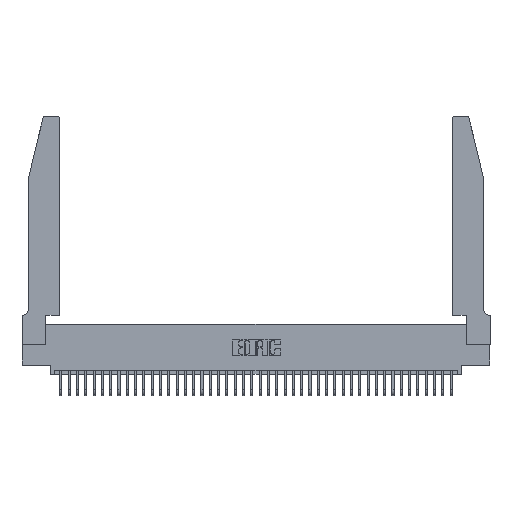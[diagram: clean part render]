
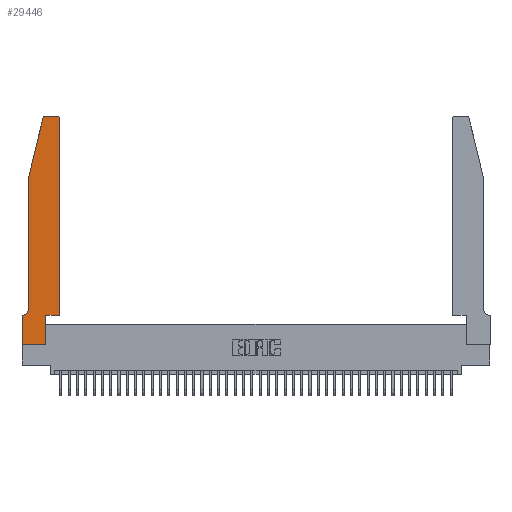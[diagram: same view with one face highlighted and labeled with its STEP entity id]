
A CAD part, top view. The second image highlights one B-rep face of the part: STEP entity #29446.
In plain terms, the highlighted planar face has unit normal (0, 0, 1).
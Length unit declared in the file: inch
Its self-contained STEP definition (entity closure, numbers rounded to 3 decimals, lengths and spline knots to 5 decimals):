
#375 = AXIS2_PLACEMENT_3D ( 'NONE', #7597, #30998, #10996 ) ;
#443 = VERTEX_POINT ( 'NONE', #25061 ) ;
#1392 = CIRCLE ( 'NONE', #7124, 0.03 ) ;
#1863 = ORIENTED_EDGE ( 'NONE', *, *, #19741, .T. ) ;
#1876 = FACE_OUTER_BOUND ( 'NONE', #27281, .T. ) ;
#3593 = LINE ( 'NONE', #36988, #31381 ) ;
#3890 = VECTOR ( 'NONE', #8353, 39.37008 ) ;
#4592 = CARTESIAN_POINT ( 'NONE',  ( 0.284, 2.75, 0.37 ) ) ;
#4842 = EDGE_CURVE ( 'NONE', #22858, #41574, #39534, .T. ) ;
#6413 = VECTOR ( 'NONE', #42172, 39.37008 ) ;
#7063 = ORIENTED_EDGE ( 'NONE', *, *, #30207, .T. ) ;
#7124 = AXIS2_PLACEMENT_3D ( 'NONE', #10562, #33948, #13940 ) ;
#7597 = CARTESIAN_POINT ( 'NONE',  ( 0.0055, 0.42, 0.37 ) ) ;
#8353 = DIRECTION ( 'NONE',  ( -0.239, -0.971, 0. ) ) ;
#8403 = DIRECTION ( 'NONE',  ( 0., 1., 0. ) ) ;
#8424 = DIRECTION ( 'NONE',  ( 0., -1., 0. ) ) ;
#9290 = CARTESIAN_POINT ( 'NONE',  ( 0., 0.35, 0.37 ) ) ;
#9339 = EDGE_CURVE ( 'NONE', #443, #17640, #28686, .T. ) ;
#10196 = VERTEX_POINT ( 'NONE', #34049 ) ;
#10318 = CARTESIAN_POINT ( 'NONE',  ( 0.284, 2.72, 0.37 ) ) ;
#10562 = CARTESIAN_POINT ( 'NONE',  ( 0.4205, 2.72, 0.37 ) ) ;
#10727 = CARTESIAN_POINT ( 'NONE',  ( 0., 0., 0.37 ) ) ;
#10894 = VECTOR ( 'NONE', #42439, 39.37008 ) ;
#10996 = DIRECTION ( 'NONE',  ( -1., 0., 0. ) ) ;
#12201 = DIRECTION ( 'NONE',  ( 1., 0., 0. ) ) ;
#13354 = ORIENTED_EDGE ( 'NONE', *, *, #23397, .T. ) ;
#13368 = LINE ( 'NONE', #19844, #20181 ) ;
#13381 = VERTEX_POINT ( 'NONE', #36469 ) ;
#13696 = DIRECTION ( 'NONE',  ( 1., 0., 0. ) ) ;
#13940 = DIRECTION ( 'NONE',  ( 1., 0., 0. ) ) ;
#14073 = ORIENTED_EDGE ( 'NONE', *, *, #34674, .T. ) ;
#15344 = EDGE_CURVE ( 'NONE', #24610, #22028, #13368, .T. ) ;
#15837 = ORIENTED_EDGE ( 'NONE', *, *, #17032, .T. ) ;
#16259 = VECTOR ( 'NONE', #12201, 39.37008 ) ;
#16424 = DIRECTION ( 'NONE',  ( 0., 0., 1. ) ) ;
#16578 = VERTEX_POINT ( 'NONE', #43088 ) ;
#17032 = EDGE_CURVE ( 'NONE', #41574, #16578, #24220, .T. ) ;
#17319 = LINE ( 'NONE', #22134, #16259 ) ;
#17443 = CIRCLE ( 'NONE', #375, 0.07 ) ;
#17640 = VERTEX_POINT ( 'NONE', #9290 ) ;
#19472 = EDGE_CURVE ( 'NONE', #10196, #42758, #27251, .T. ) ;
#19741 = EDGE_CURVE ( 'NONE', #40538, #22858, #34519, .T. ) ;
#19765 = CARTESIAN_POINT ( 'NONE',  ( 0.4505, 2.72, 0.37 ) ) ;
#19844 = CARTESIAN_POINT ( 'NONE',  ( 0.4505, 0.35, 0.37 ) ) ;
#20168 = DIRECTION ( 'NONE',  ( -1., 0., 0. ) ) ;
#20181 = VECTOR ( 'NONE', #36484, 39.37008 ) ;
#20415 = EDGE_CURVE ( 'NONE', #22028, #13381, #1392, .T. ) ;
#22028 = VERTEX_POINT ( 'NONE', #19765 ) ;
#22134 = CARTESIAN_POINT ( 'NONE',  ( 0., 0., 0.37 ) ) ;
#22150 = CARTESIAN_POINT ( 'NONE',  ( 0.0755, 2., 0.37 ) ) ;
#22830 = VECTOR ( 'NONE', #20168, 39.37008 ) ;
#22858 = VERTEX_POINT ( 'NONE', #30448 ) ;
#22919 = ORIENTED_EDGE ( 'NONE', *, *, #31930, .T. ) ;
#23197 = CARTESIAN_POINT ( 'NONE',  ( 0.2605, 2.75, 0.37 ) ) ;
#23397 = EDGE_CURVE ( 'NONE', #16578, #443, #17443, .T. ) ;
#24220 = LINE ( 'NONE', #22150, #6413 ) ;
#24610 = VERTEX_POINT ( 'NONE', #34712 ) ;
#24782 = EDGE_CURVE ( 'NONE', #34089, #10196, #17319, .T. ) ;
#25061 = CARTESIAN_POINT ( 'NONE',  ( 0.0055, 0.35, 0.37 ) ) ;
#25076 = CARTESIAN_POINT ( 'NONE',  ( 0.2865, 0.35, 0.37 ) ) ;
#25358 = LINE ( 'NONE', #31817, #35298 ) ;
#25763 = CARTESIAN_POINT ( 'NONE',  ( 0.0755, 0.35, 0.37 ) ) ;
#26175 = CARTESIAN_POINT ( 'NONE',  ( 0.0755, 2., 0.37 ) ) ;
#27251 = LINE ( 'NONE', #25076, #35061 ) ;
#27281 = EDGE_LOOP ( 'NONE', ( #7063, #1863, #34715, #15837, #13354, #32390, #22919, #36992, #31744, #14073, #41542, #33229 ) ) ;
#28686 = LINE ( 'NONE', #25763, #10894 ) ;
#29446 = ADVANCED_FACE ( 'NONE', ( #1876 ), #29543, .T. ) ;
#29543 = PLANE ( 'NONE',  #31147 ) ;
#30207 = EDGE_CURVE ( 'NONE', #13381, #40538, #31711, .T. ) ;
#30448 = CARTESIAN_POINT ( 'NONE',  ( 0.25487, 2.72718, 0.37 ) ) ;
#30998 = DIRECTION ( 'NONE',  ( 0., 0., -1. ) ) ;
#31147 = AXIS2_PLACEMENT_3D ( 'NONE', #36431, #16424, #39782 ) ;
#31381 = VECTOR ( 'NONE', #40333, 39.37008 ) ;
#31711 = LINE ( 'NONE', #23197, #22830 ) ;
#31744 = ORIENTED_EDGE ( 'NONE', *, *, #19472, .T. ) ;
#31750 = CARTESIAN_POINT ( 'NONE',  ( 0.0755, 2., 0.37 ) ) ;
#31817 = CARTESIAN_POINT ( 'NONE',  ( 0., 0., 0.37 ) ) ;
#31930 = EDGE_CURVE ( 'NONE', #17640, #34089, #25358, .T. ) ;
#32057 = AXIS2_PLACEMENT_3D ( 'NONE', #10318, #33720, #13696 ) ;
#32390 = ORIENTED_EDGE ( 'NONE', *, *, #9339, .T. ) ;
#33229 = ORIENTED_EDGE ( 'NONE', *, *, #20415, .T. ) ;
#33720 = DIRECTION ( 'NONE',  ( 0., 0., 1. ) ) ;
#33948 = DIRECTION ( 'NONE',  ( 0., 0., 1. ) ) ;
#34049 = CARTESIAN_POINT ( 'NONE',  ( 0.2865, 0., 0.37 ) ) ;
#34089 = VERTEX_POINT ( 'NONE', #10727 ) ;
#34519 = CIRCLE ( 'NONE', #32057, 0.03 ) ;
#34674 = EDGE_CURVE ( 'NONE', #42758, #24610, #3593, .T. ) ;
#34712 = CARTESIAN_POINT ( 'NONE',  ( 0.4505, 0.35, 0.37 ) ) ;
#34715 = ORIENTED_EDGE ( 'NONE', *, *, #4842, .T. ) ;
#35061 = VECTOR ( 'NONE', #8403, 39.37008 ) ;
#35298 = VECTOR ( 'NONE', #8424, 39.37008 ) ;
#36431 = CARTESIAN_POINT ( 'NONE',  ( 0., 0.35, 0.37 ) ) ;
#36469 = CARTESIAN_POINT ( 'NONE',  ( 0.4205, 2.75, 0.37 ) ) ;
#36484 = DIRECTION ( 'NONE',  ( 0., 1., 0. ) ) ;
#36988 = CARTESIAN_POINT ( 'NONE',  ( 0.4505, 0.35, 0.37 ) ) ;
#36992 = ORIENTED_EDGE ( 'NONE', *, *, #24782, .T. ) ;
#39534 = LINE ( 'NONE', #31750, #3890 ) ;
#39782 = DIRECTION ( 'NONE',  ( 1., 0., 0. ) ) ;
#40333 = DIRECTION ( 'NONE',  ( 1., 0., 0. ) ) ;
#40538 = VERTEX_POINT ( 'NONE', #4592 ) ;
#41542 = ORIENTED_EDGE ( 'NONE', *, *, #15344, .T. ) ;
#41574 = VERTEX_POINT ( 'NONE', #26175 ) ;
#41869 = CARTESIAN_POINT ( 'NONE',  ( 0.2865, 0.35, 0.37 ) ) ;
#42172 = DIRECTION ( 'NONE',  ( 0., -1., 0. ) ) ;
#42439 = DIRECTION ( 'NONE',  ( -1., 0., 0. ) ) ;
#42758 = VERTEX_POINT ( 'NONE', #41869 ) ;
#43088 = CARTESIAN_POINT ( 'NONE',  ( 0.0755, 0.42, 0.37 ) ) ;
